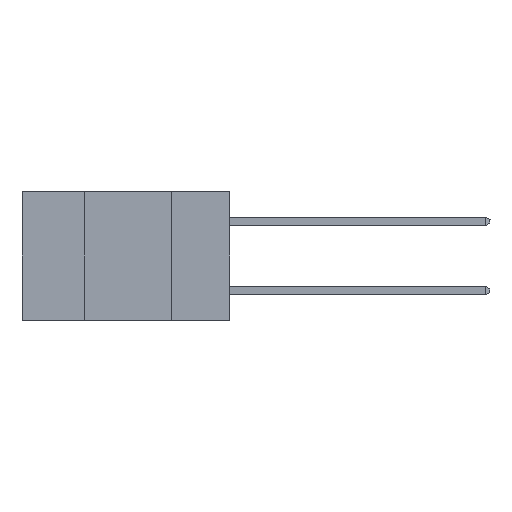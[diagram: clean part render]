
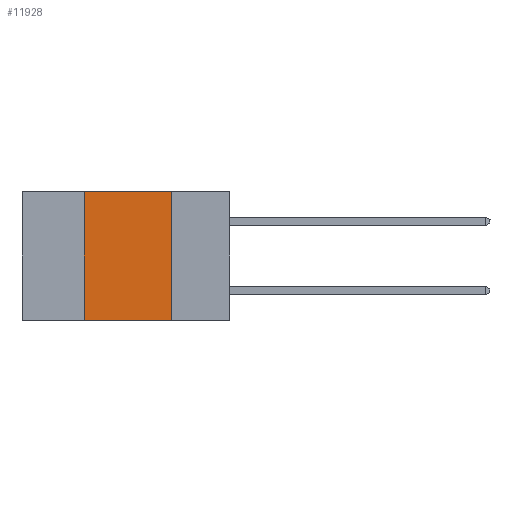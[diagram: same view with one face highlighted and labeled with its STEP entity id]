
A CAD part, left-side view. The second image highlights one B-rep face of the part: STEP entity #11928.
In plain terms, the highlighted planar face has unit normal (-1, 0, 0).
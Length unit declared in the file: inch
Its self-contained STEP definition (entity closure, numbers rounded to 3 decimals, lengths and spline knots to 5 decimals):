
#7 = DIRECTION ( 'NONE',  ( 0., 0., 1. ) ) ;
#766 = DIRECTION ( 'NONE',  ( 0., -1., 0. ) ) ;
#1033 = CARTESIAN_POINT ( 'NONE',  ( 0., 0.42, -0.37 ) ) ;
#1071 = VERTEX_POINT ( 'NONE', #11569 ) ;
#1089 = VECTOR ( 'NONE', #7, 39.37008 ) ;
#1194 = VECTOR ( 'NONE', #12272, 39.37008 ) ;
#1196 = EDGE_LOOP ( 'NONE', ( #15892, #6038, #15100, #1865 ) ) ;
#1278 = LINE ( 'NONE', #15139, #1089 ) ;
#1865 = ORIENTED_EDGE ( 'NONE', *, *, #17222, .T. ) ;
#2343 = EDGE_CURVE ( 'NONE', #5875, #1071, #1278, .T. ) ;
#2471 = VERTEX_POINT ( 'NONE', #5662 ) ;
#3184 = DIRECTION ( 'NONE',  ( 0., 0., -1. ) ) ;
#3454 = FACE_OUTER_BOUND ( 'NONE', #1196, .T. ) ;
#3706 = DIRECTION ( 'NONE',  ( 1., 0., 0. ) ) ;
#5005 = CARTESIAN_POINT ( 'NONE',  ( 0., 0.6, 0. ) ) ;
#5120 = VERTEX_POINT ( 'NONE', #17145 ) ;
#5226 = EDGE_CURVE ( 'NONE', #2471, #5120, #13108, .T. ) ;
#5662 = CARTESIAN_POINT ( 'NONE',  ( 0., 0.17, 0. ) ) ;
#5875 = VERTEX_POINT ( 'NONE', #1033 ) ;
#6038 = ORIENTED_EDGE ( 'NONE', *, *, #8590, .F. ) ;
#6479 = CARTESIAN_POINT ( 'NONE',  ( 0., 0.6, 0. ) ) ;
#6662 = VECTOR ( 'NONE', #766, 39.37008 ) ;
#7697 = AXIS2_PLACEMENT_3D ( 'NONE', #6479, #3706, #9310 ) ;
#8075 = CARTESIAN_POINT ( 'NONE',  ( 0., 0.6, -0.37 ) ) ;
#8590 = EDGE_CURVE ( 'NONE', #1071, #2471, #17601, .T. ) ;
#9310 = DIRECTION ( 'NONE',  ( 0., 0., -1. ) ) ;
#10168 = CARTESIAN_POINT ( 'NONE',  ( 0., 0.17, -0.37 ) ) ;
#10639 = PLANE ( 'NONE',  #7697 ) ;
#10768 = LINE ( 'NONE', #8075, #6662 ) ;
#11569 = CARTESIAN_POINT ( 'NONE',  ( 0., 0.42, 0. ) ) ;
#11928 = ADVANCED_FACE ( 'NONE', ( #3454 ), #10639, .F. ) ;
#12250 = VECTOR ( 'NONE', #3184, 39.37008 ) ;
#12272 = DIRECTION ( 'NONE',  ( 0., -1., 0. ) ) ;
#13108 = LINE ( 'NONE', #10168, #12250 ) ;
#15100 = ORIENTED_EDGE ( 'NONE', *, *, #2343, .F. ) ;
#15139 = CARTESIAN_POINT ( 'NONE',  ( 0., 0.42, -0.37 ) ) ;
#15892 = ORIENTED_EDGE ( 'NONE', *, *, #5226, .F. ) ;
#17145 = CARTESIAN_POINT ( 'NONE',  ( 0., 0.17, -0.37 ) ) ;
#17222 = EDGE_CURVE ( 'NONE', #5875, #5120, #10768, .T. ) ;
#17601 = LINE ( 'NONE', #5005, #1194 ) ;
